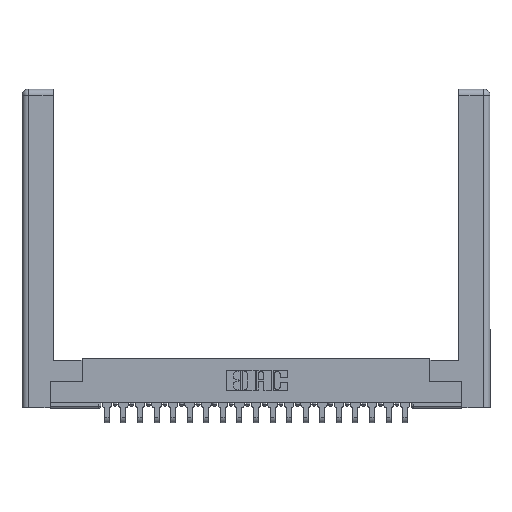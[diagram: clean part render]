
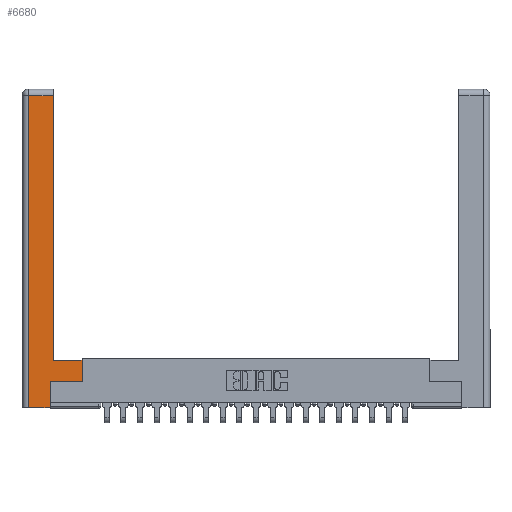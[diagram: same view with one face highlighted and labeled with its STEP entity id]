
A CAD part, top view. The second image highlights one B-rep face of the part: STEP entity #6680.
In plain terms, the highlighted planar face has unit normal (0, 0, 1).
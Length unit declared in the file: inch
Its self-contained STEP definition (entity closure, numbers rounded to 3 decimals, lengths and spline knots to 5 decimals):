
#7 = LINE ( 'NONE', #11168, #6905 ) ;
#113 = LINE ( 'NONE', #13934, #3567 ) ;
#633 = VERTEX_POINT ( 'NONE', #8377 ) ;
#889 = CARTESIAN_POINT ( 'NONE',  ( 0.295, 2.94, 0. ) ) ;
#1839 = VERTEX_POINT ( 'NONE', #889 ) ;
#2415 = PLANE ( 'NONE',  #5122 ) ;
#2542 = EDGE_CURVE ( 'NONE', #12932, #10844, #16298, .T. ) ;
#3183 = LINE ( 'NONE', #19428, #16072 ) ;
#3441 = LINE ( 'NONE', #4358, #16311 ) ;
#3567 = VECTOR ( 'NONE', #12371, 39.37008 ) ;
#4028 = FACE_OUTER_BOUND ( 'NONE', #19402, .T. ) ;
#4358 = CARTESIAN_POINT ( 'NONE',  ( 0.265, 0.245, 0. ) ) ;
#5050 = ORIENTED_EDGE ( 'NONE', *, *, #8975, .T. ) ;
#5122 = AXIS2_PLACEMENT_3D ( 'NONE', #14232, #17730, #12609 ) ;
#5153 = CARTESIAN_POINT ( 'NONE',  ( 0.295, 0.45, 0. ) ) ;
#5187 = ORIENTED_EDGE ( 'NONE', *, *, #5268, .T. ) ;
#5249 = VERTEX_POINT ( 'NONE', #6873 ) ;
#5268 = EDGE_CURVE ( 'NONE', #19323, #1839, #113, .T. ) ;
#5427 = VECTOR ( 'NONE', #10053, 39.37008 ) ;
#6000 = LINE ( 'NONE', #21697, #14433 ) ;
#6636 = DIRECTION ( 'NONE',  ( 0., 1., 0. ) ) ;
#6672 = CARTESIAN_POINT ( 'NONE',  ( 0.265, 0., 0. ) ) ;
#6680 = ADVANCED_FACE ( 'NONE', ( #4028 ), #2415, .F. ) ;
#6873 = CARTESIAN_POINT ( 'NONE',  ( 0.0615, 2.94, 0. ) ) ;
#6905 = VECTOR ( 'NONE', #19932, 39.37008 ) ;
#7561 = EDGE_CURVE ( 'NONE', #1839, #5249, #19514, .T. ) ;
#8377 = CARTESIAN_POINT ( 'NONE',  ( 0.265, 0.245, 0. ) ) ;
#8541 = DIRECTION ( 'NONE',  ( -1., 0., 0. ) ) ;
#8975 = EDGE_CURVE ( 'NONE', #21823, #633, #3441, .T. ) ;
#9904 = LINE ( 'NONE', #20126, #5427 ) ;
#10053 = DIRECTION ( 'NONE',  ( 1., 0., 0. ) ) ;
#10342 = EDGE_CURVE ( 'NONE', #5249, #17763, #6000, .T. ) ;
#10844 = VERTEX_POINT ( 'NONE', #18475 ) ;
#11168 = CARTESIAN_POINT ( 'NONE',  ( 0.265, 0., 0. ) ) ;
#11937 = ORIENTED_EDGE ( 'NONE', *, *, #19060, .T. ) ;
#12149 = CARTESIAN_POINT ( 'NONE',  ( 0.0615, 2.94, 0. ) ) ;
#12371 = DIRECTION ( 'NONE',  ( 0., 1., 0. ) ) ;
#12609 = DIRECTION ( 'NONE',  ( -1., 0., 0. ) ) ;
#12660 = ORIENTED_EDGE ( 'NONE', *, *, #16809, .T. ) ;
#12932 = VERTEX_POINT ( 'NONE', #14276 ) ;
#13263 = CARTESIAN_POINT ( 'NONE',  ( 0.565, 0.45, 0. ) ) ;
#13934 = CARTESIAN_POINT ( 'NONE',  ( 0.295, 3., 0. ) ) ;
#14232 = CARTESIAN_POINT ( 'NONE',  ( 0., 0., 0. ) ) ;
#14276 = CARTESIAN_POINT ( 'NONE',  ( 0.565, 0.245, 0. ) ) ;
#14433 = VECTOR ( 'NONE', #16426, 39.37008 ) ;
#14603 = ORIENTED_EDGE ( 'NONE', *, *, #21012, .T. ) ;
#15056 = VECTOR ( 'NONE', #8541, 39.37008 ) ;
#16072 = VECTOR ( 'NONE', #18015, 39.37008 ) ;
#16298 = LINE ( 'NONE', #13263, #21600 ) ;
#16299 = ORIENTED_EDGE ( 'NONE', *, *, #10342, .T. ) ;
#16311 = VECTOR ( 'NONE', #17820, 39.37008 ) ;
#16426 = DIRECTION ( 'NONE',  ( 0., -1., 0. ) ) ;
#16809 = EDGE_CURVE ( 'NONE', #633, #12932, #9904, .T. ) ;
#17716 = ORIENTED_EDGE ( 'NONE', *, *, #7561, .T. ) ;
#17718 = ORIENTED_EDGE ( 'NONE', *, *, #2542, .T. ) ;
#17730 = DIRECTION ( 'NONE',  ( 0., 0., -1. ) ) ;
#17763 = VERTEX_POINT ( 'NONE', #19770 ) ;
#17820 = DIRECTION ( 'NONE',  ( 0., 1., 0. ) ) ;
#18015 = DIRECTION ( 'NONE',  ( -1., 0., 0. ) ) ;
#18475 = CARTESIAN_POINT ( 'NONE',  ( 0.565, 0.45, 0. ) ) ;
#19060 = EDGE_CURVE ( 'NONE', #10844, #19323, #3183, .T. ) ;
#19323 = VERTEX_POINT ( 'NONE', #5153 ) ;
#19402 = EDGE_LOOP ( 'NONE', ( #5187, #17716, #16299, #14603, #5050, #12660, #17718, #11937 ) ) ;
#19428 = CARTESIAN_POINT ( 'NONE',  ( 0.295, 0.45, 0. ) ) ;
#19514 = LINE ( 'NONE', #12149, #15056 ) ;
#19770 = CARTESIAN_POINT ( 'NONE',  ( 0.0615, 0., 0. ) ) ;
#19932 = DIRECTION ( 'NONE',  ( 1., 0., 0. ) ) ;
#20126 = CARTESIAN_POINT ( 'NONE',  ( 0.565, 0.245, 0. ) ) ;
#21012 = EDGE_CURVE ( 'NONE', #17763, #21823, #7, .T. ) ;
#21600 = VECTOR ( 'NONE', #6636, 39.37008 ) ;
#21697 = CARTESIAN_POINT ( 'NONE',  ( 0.0615, 0., 0. ) ) ;
#21823 = VERTEX_POINT ( 'NONE', #6672 ) ;
